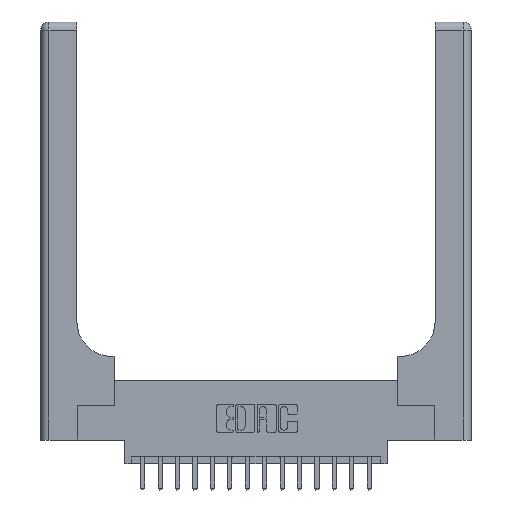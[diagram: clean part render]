
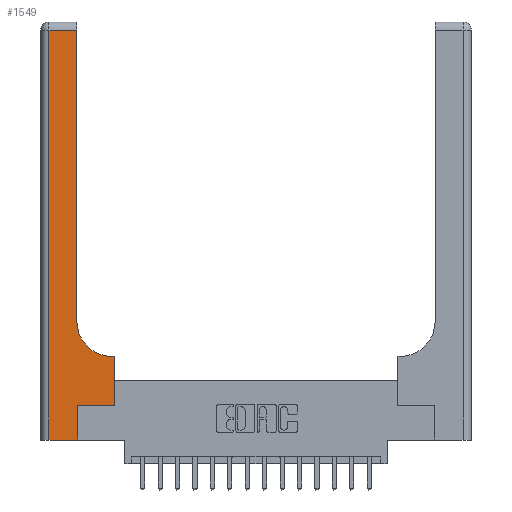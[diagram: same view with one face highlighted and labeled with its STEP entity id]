
A CAD part, top view. The second image highlights one B-rep face of the part: STEP entity #1549.
In plain terms, the highlighted planar face has unit normal (0, 0, 1).
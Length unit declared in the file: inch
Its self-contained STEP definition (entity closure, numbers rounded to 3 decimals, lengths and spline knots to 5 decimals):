
#65 = VERTEX_POINT ( 'NONE', #1366 ) ;
#137 = VECTOR ( 'NONE', #4729, 39.37008 ) ;
#281 = ORIENTED_EDGE ( 'NONE', *, *, #12337, .T. ) ;
#706 = ORIENTED_EDGE ( 'NONE', *, *, #12025, .T. ) ;
#1206 = CIRCLE ( 'NONE', #6616, 0.25 ) ;
#1271 = CARTESIAN_POINT ( 'NONE',  ( 0.26, 2.94, 0.37 ) ) ;
#1366 = CARTESIAN_POINT ( 'NONE',  ( 0.528, 0.6, 0.37 ) ) ;
#1549 = ADVANCED_FACE ( 'NONE', ( #17542 ), #8995, .F. ) ;
#1824 = VECTOR ( 'NONE', #5816, 39.37008 ) ;
#1926 = CARTESIAN_POINT ( 'NONE',  ( 0.06, 0., 0.37 ) ) ;
#2410 = VECTOR ( 'NONE', #10747, 39.37008 ) ;
#2430 = VECTOR ( 'NONE', #13008, 39.37008 ) ;
#2695 = VERTEX_POINT ( 'NONE', #1926 ) ;
#2725 = CARTESIAN_POINT ( 'NONE',  ( 0.06, 2.94, 0.37 ) ) ;
#2911 = CARTESIAN_POINT ( 'NONE',  ( 0.26, 3., 0.37 ) ) ;
#3187 = EDGE_CURVE ( 'NONE', #65, #15957, #12634, .T. ) ;
#3241 = ORIENTED_EDGE ( 'NONE', *, *, #14756, .T. ) ;
#3557 = EDGE_CURVE ( 'NONE', #15060, #65, #10207, .T. ) ;
#3751 = CARTESIAN_POINT ( 'NONE',  ( 0., 3., 0.37 ) ) ;
#3888 = CARTESIAN_POINT ( 'NONE',  ( 0.26, 0.6, 0.37 ) ) ;
#3935 = ORIENTED_EDGE ( 'NONE', *, *, #3187, .T. ) ;
#4126 = EDGE_CURVE ( 'NONE', #13752, #15060, #5957, .T. ) ;
#4729 = DIRECTION ( 'NONE',  ( -1., 0., 0. ) ) ;
#5044 = VERTEX_POINT ( 'NONE', #1271 ) ;
#5693 = LINE ( 'NONE', #11200, #9533 ) ;
#5775 = DIRECTION ( 'NONE',  ( 0., 1., 0. ) ) ;
#5803 = CARTESIAN_POINT ( 'NONE',  ( 0.265, 0.25, 0.37 ) ) ;
#5816 = DIRECTION ( 'NONE',  ( 1., 0., 0. ) ) ;
#5957 = LINE ( 'NONE', #10467, #2410 ) ;
#6415 = DIRECTION ( 'NONE',  ( 0., 1., 0. ) ) ;
#6441 = VECTOR ( 'NONE', #5775, 39.37008 ) ;
#6616 = AXIS2_PLACEMENT_3D ( 'NONE', #16262, #8036, #17605 ) ;
#6680 = CARTESIAN_POINT ( 'NONE',  ( 0.528, 0.25, 0.37 ) ) ;
#6692 = CARTESIAN_POINT ( 'NONE',  ( 0., 2.94, 0.37 ) ) ;
#7502 = LINE ( 'NONE', #10684, #11220 ) ;
#8036 = DIRECTION ( 'NONE',  ( 0., 0., -1. ) ) ;
#8290 = ORIENTED_EDGE ( 'NONE', *, *, #3557, .T. ) ;
#8971 = ORIENTED_EDGE ( 'NONE', *, *, #11151, .T. ) ;
#8995 = PLANE ( 'NONE',  #13228 ) ;
#9141 = CARTESIAN_POINT ( 'NONE',  ( 0.26, 0.85, 0.37 ) ) ;
#9279 = VERTEX_POINT ( 'NONE', #9141 ) ;
#9533 = VECTOR ( 'NONE', #12603, 39.37008 ) ;
#9899 = VERTEX_POINT ( 'NONE', #2725 ) ;
#10207 = LINE ( 'NONE', #6680, #6441 ) ;
#10467 = CARTESIAN_POINT ( 'NONE',  ( 0.265, 0.25, 0.37 ) ) ;
#10521 = LINE ( 'NONE', #18224, #1824 ) ;
#10684 = CARTESIAN_POINT ( 'NONE',  ( 0.265, 0., 0.37 ) ) ;
#10747 = DIRECTION ( 'NONE',  ( 1., 0., 0. ) ) ;
#10804 = EDGE_LOOP ( 'NONE', ( #281, #706, #13031, #8971, #17048, #17838, #8290, #3935, #3241 ) ) ;
#11151 = EDGE_CURVE ( 'NONE', #2695, #13943, #10521, .T. ) ;
#11200 = CARTESIAN_POINT ( 'NONE',  ( 0.06, 3., 0.37 ) ) ;
#11220 = VECTOR ( 'NONE', #6415, 39.37008 ) ;
#11362 = CARTESIAN_POINT ( 'NONE',  ( 0.528, 0.25, 0.37 ) ) ;
#12025 = EDGE_CURVE ( 'NONE', #5044, #9899, #13703, .T. ) ;
#12337 = EDGE_CURVE ( 'NONE', #9279, #5044, #17069, .T. ) ;
#12603 = DIRECTION ( 'NONE',  ( 0., -1., 0. ) ) ;
#12634 = LINE ( 'NONE', #3888, #137 ) ;
#12934 = CARTESIAN_POINT ( 'NONE',  ( 0.51, 0.6, 0.37 ) ) ;
#12974 = DIRECTION ( 'NONE',  ( 0., 0., -1. ) ) ;
#13008 = DIRECTION ( 'NONE',  ( 0., 1., 0. ) ) ;
#13031 = ORIENTED_EDGE ( 'NONE', *, *, #14287, .T. ) ;
#13228 = AXIS2_PLACEMENT_3D ( 'NONE', #3751, #12974, #14384 ) ;
#13703 = LINE ( 'NONE', #6692, #16497 ) ;
#13752 = VERTEX_POINT ( 'NONE', #5803 ) ;
#13943 = VERTEX_POINT ( 'NONE', #14532 ) ;
#14287 = EDGE_CURVE ( 'NONE', #9899, #2695, #5693, .T. ) ;
#14384 = DIRECTION ( 'NONE',  ( -1., 0., 0. ) ) ;
#14532 = CARTESIAN_POINT ( 'NONE',  ( 0.265, 0., 0.37 ) ) ;
#14756 = EDGE_CURVE ( 'NONE', #15957, #9279, #1206, .T. ) ;
#15060 = VERTEX_POINT ( 'NONE', #11362 ) ;
#15583 = EDGE_CURVE ( 'NONE', #13943, #13752, #7502, .T. ) ;
#15957 = VERTEX_POINT ( 'NONE', #12934 ) ;
#16262 = CARTESIAN_POINT ( 'NONE',  ( 0.51, 0.85, 0.37 ) ) ;
#16497 = VECTOR ( 'NONE', #17730, 39.37008 ) ;
#17048 = ORIENTED_EDGE ( 'NONE', *, *, #15583, .T. ) ;
#17069 = LINE ( 'NONE', #2911, #2430 ) ;
#17542 = FACE_OUTER_BOUND ( 'NONE', #10804, .T. ) ;
#17605 = DIRECTION ( 'NONE',  ( 1., 0., 0. ) ) ;
#17730 = DIRECTION ( 'NONE',  ( -1., 0., 0. ) ) ;
#17838 = ORIENTED_EDGE ( 'NONE', *, *, #4126, .T. ) ;
#18224 = CARTESIAN_POINT ( 'NONE',  ( 0., 0., 0.37 ) ) ;
